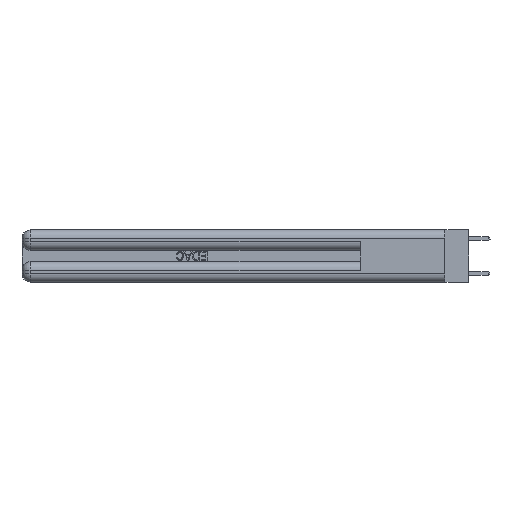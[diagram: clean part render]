
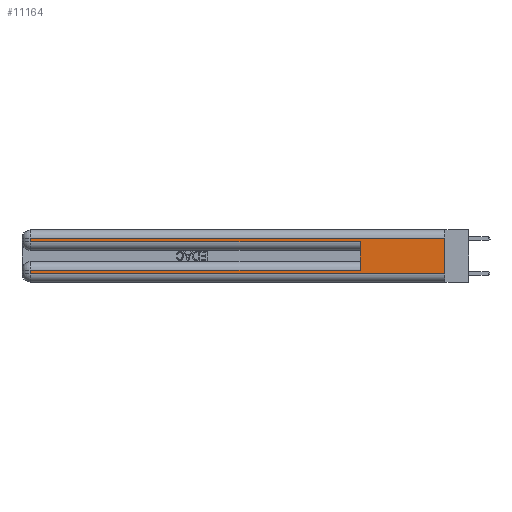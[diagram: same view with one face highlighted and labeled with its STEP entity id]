
A CAD part, left-side view. The second image highlights one B-rep face of the part: STEP entity #11164.
In plain terms, the highlighted planar face has unit normal (-1, 0, 0).
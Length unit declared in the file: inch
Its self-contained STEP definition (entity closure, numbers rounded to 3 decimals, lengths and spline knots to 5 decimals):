
#335 = ORIENTED_EDGE ( 'NONE', *, *, #6089, .F. ) ;
#773 = VERTEX_POINT ( 'NONE', #16735 ) ;
#785 = CARTESIAN_POINT ( 'NONE',  ( 0., 0., 0.06 ) ) ;
#944 = ORIENTED_EDGE ( 'NONE', *, *, #6397, .T. ) ;
#1213 = CARTESIAN_POINT ( 'NONE',  ( 0., 0.6, 0.085 ) ) ;
#1276 = VERTEX_POINT ( 'NONE', #24159 ) ;
#1350 = CARTESIAN_POINT ( 'NONE',  ( 0., 2.94, 0.285 ) ) ;
#1433 = EDGE_CURVE ( 'NONE', #18605, #18848, #21233, .T. ) ;
#2043 = VERTEX_POINT ( 'NONE', #6553 ) ;
#3447 = ORIENTED_EDGE ( 'NONE', *, *, #1433, .T. ) ;
#3518 = CARTESIAN_POINT ( 'NONE',  ( 0., 2.94, 0.06 ) ) ;
#4084 = ORIENTED_EDGE ( 'NONE', *, *, #10269, .T. ) ;
#4085 = EDGE_CURVE ( 'NONE', #25910, #773, #21452, .T. ) ;
#4555 = CARTESIAN_POINT ( 'NONE',  ( 0., 0., 0.31 ) ) ;
#5589 = CARTESIAN_POINT ( 'NONE',  ( 0., 0., 0.37 ) ) ;
#5729 = VECTOR ( 'NONE', #15389, 39.37008 ) ;
#5733 = PLANE ( 'NONE',  #25593 ) ;
#6089 = EDGE_CURVE ( 'NONE', #25910, #1276, #11275, .T. ) ;
#6333 = VERTEX_POINT ( 'NONE', #3518 ) ;
#6397 = EDGE_CURVE ( 'NONE', #21657, #1276, #19115, .T. ) ;
#6553 = CARTESIAN_POINT ( 'NONE',  ( 0., 0., 0.06 ) ) ;
#6588 = DIRECTION ( 'NONE',  ( 0., 1., 0. ) ) ;
#6864 = ORIENTED_EDGE ( 'NONE', *, *, #20187, .F. ) ;
#6950 = CARTESIAN_POINT ( 'NONE',  ( 0., 0., 0.085 ) ) ;
#6958 = DIRECTION ( 'NONE',  ( 0., -1., 0. ) ) ;
#7792 = DIRECTION ( 'NONE',  ( 1., 0., 0. ) ) ;
#8461 = VECTOR ( 'NONE', #11781, 39.37008 ) ;
#8927 = DIRECTION ( 'NONE',  ( 0., 0., 1. ) ) ;
#10101 = VECTOR ( 'NONE', #21033, 39.37008 ) ;
#10269 = EDGE_CURVE ( 'NONE', #18848, #21657, #13290, .T. ) ;
#11164 = ADVANCED_FACE ( 'NONE', ( #13882 ), #5733, .F. ) ;
#11275 = LINE ( 'NONE', #12919, #16627 ) ;
#11353 = CARTESIAN_POINT ( 'NONE',  ( 0., 2.94, 0.37 ) ) ;
#11781 = DIRECTION ( 'NONE',  ( 0., -1., 0. ) ) ;
#12229 = ORIENTED_EDGE ( 'NONE', *, *, #4085, .T. ) ;
#12768 = CARTESIAN_POINT ( 'NONE',  ( 0., 2.94, 0.31 ) ) ;
#12919 = CARTESIAN_POINT ( 'NONE',  ( 0., 0.6, 0.145 ) ) ;
#13290 = LINE ( 'NONE', #18961, #23386 ) ;
#13794 = CARTESIAN_POINT ( 'NONE',  ( 0., 0., 0.285 ) ) ;
#13882 = FACE_OUTER_BOUND ( 'NONE', #17519, .T. ) ;
#15225 = VECTOR ( 'NONE', #6588, 39.37008 ) ;
#15389 = DIRECTION ( 'NONE',  ( 0., 0., -1. ) ) ;
#15879 = EDGE_CURVE ( 'NONE', #773, #6333, #21170, .T. ) ;
#16180 = ORIENTED_EDGE ( 'NONE', *, *, #15879, .T. ) ;
#16627 = VECTOR ( 'NONE', #8927, 39.37008 ) ;
#16735 = CARTESIAN_POINT ( 'NONE',  ( 0., 2.94, 0.085 ) ) ;
#16946 = DIRECTION ( 'NONE',  ( 0., 0., -1. ) ) ;
#17519 = EDGE_LOOP ( 'NONE', ( #6864, #3447, #4084, #944, #335, #12229, #16180, #19723 ) ) ;
#18605 = VERTEX_POINT ( 'NONE', #22067 ) ;
#18848 = VERTEX_POINT ( 'NONE', #12768 ) ;
#18961 = CARTESIAN_POINT ( 'NONE',  ( 0., 2.94, 0.37 ) ) ;
#19115 = LINE ( 'NONE', #13794, #8461 ) ;
#19723 = ORIENTED_EDGE ( 'NONE', *, *, #21489, .T. ) ;
#19970 = LINE ( 'NONE', #785, #24010 ) ;
#20187 = EDGE_CURVE ( 'NONE', #18605, #2043, #22860, .T. ) ;
#21033 = DIRECTION ( 'NONE',  ( 0., 1., 0. ) ) ;
#21170 = LINE ( 'NONE', #11353, #5729 ) ;
#21233 = LINE ( 'NONE', #4555, #15225 ) ;
#21452 = LINE ( 'NONE', #6950, #10101 ) ;
#21489 = EDGE_CURVE ( 'NONE', #6333, #2043, #19970, .T. ) ;
#21657 = VERTEX_POINT ( 'NONE', #1350 ) ;
#21878 = DIRECTION ( 'NONE',  ( 0., 0., -1. ) ) ;
#22067 = CARTESIAN_POINT ( 'NONE',  ( 0., 0., 0.31 ) ) ;
#22244 = VECTOR ( 'NONE', #23712, 39.37008 ) ;
#22860 = LINE ( 'NONE', #5589, #22244 ) ;
#23386 = VECTOR ( 'NONE', #16946, 39.37008 ) ;
#23712 = DIRECTION ( 'NONE',  ( 0., 0., -1. ) ) ;
#23763 = CARTESIAN_POINT ( 'NONE',  ( 0., 0., 0.37 ) ) ;
#24010 = VECTOR ( 'NONE', #6958, 39.37008 ) ;
#24159 = CARTESIAN_POINT ( 'NONE',  ( 0., 0.6, 0.285 ) ) ;
#25593 = AXIS2_PLACEMENT_3D ( 'NONE', #23763, #7792, #21878 ) ;
#25910 = VERTEX_POINT ( 'NONE', #1213 ) ;
